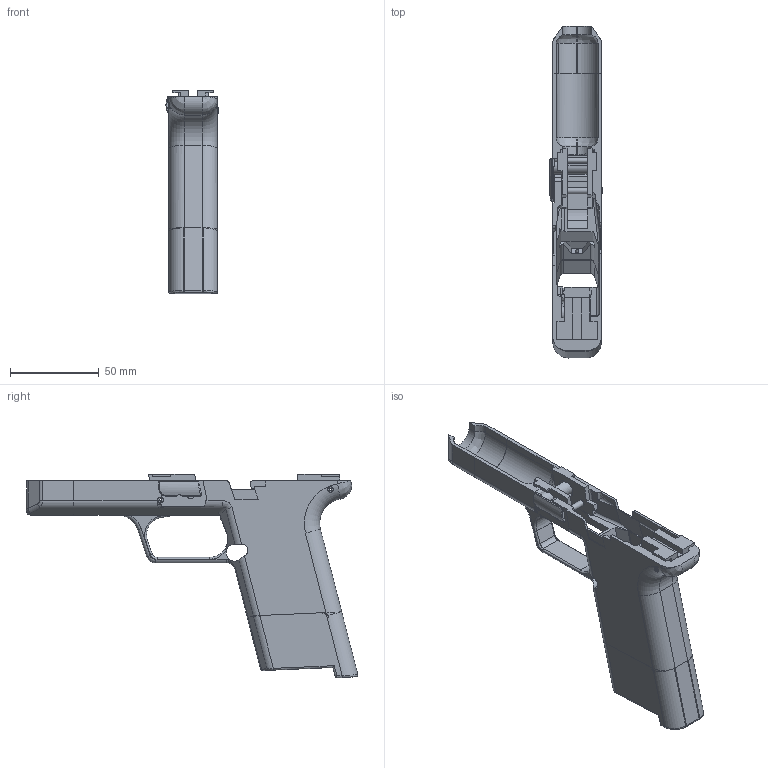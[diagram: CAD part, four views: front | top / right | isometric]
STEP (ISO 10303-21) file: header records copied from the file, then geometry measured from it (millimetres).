
FILE_DESCRIPTION(/* description */ (''),/* implementation_level */ '2;1');
FILE_NAME(/* name */ 'M&P 9 Assembly.step',/* time_stamp */ '2021-05-28T01:57:19-04:00',/* author */ (''),/* organization */ (''),/* preprocessor_version */ 'ST-DEVELOPER v18.1',/* originating_system */ 'Autodesk Translation Framework v10.6.0.1341',/* authorisation */ '');
FILE_SCHEMA (('AUTOMOTIVE_DESIGN { 1 0 10303 214 3 1 1 }'));
Length unit declared in the file: millimetre
Products named in the file (11): M&P 9 Reference; Rear Fire Control Group Pin; Front Locking Block Group Pin; Trigger Pin; Locking Block; Disassembly Lug; Rear Fire Control Group; Frame; Fitment Section; Nose; Full-Size Magwell Body
Assembly tree (10 placements, depth 4):
  M&P 9 Reference
    Rear Fire Control Group Pin
    Front Locking Block Group Pin
    Trigger Pin
    Locking Block
    Disassembly Lug
    Rear Fire Control Group
    Frame
      Fitment Section
        Nose
      Full-Size Magwell Body
Bounding box: 29.39 x 187.16 x 114.81 mm (x, y, z)
Volume: 102131.5 mm3; surface area: 56637.7 mm2
Topology: 11 solids, 11 shells, 544 faces, 1479 edges, 942 vertices
Faces by surface type: plane 281, cylinder 171, bspline 68, torus 17, sphere 6, cone 1
Full cylindrical faces by diameter (mm): 1.35 x2, 2 x3, 3.15 x2, 3.18 x3, 3.2 x2, 3.361 x2, 3.5 x1, 3.55 x4, 4.7 x1, 6.3 x1, 7.7 x1, 8.8 x1, 9 x2
Entity records: 19638 total; most frequent: CARTESIAN_POINT 5589, ORIENTED_EDGE 2950, DIRECTION 2794, EDGE_CURVE 1475, VERTEX_POINT 942, AXIS2_PLACEMENT_3D 937, LINE 920, VECTOR 920
